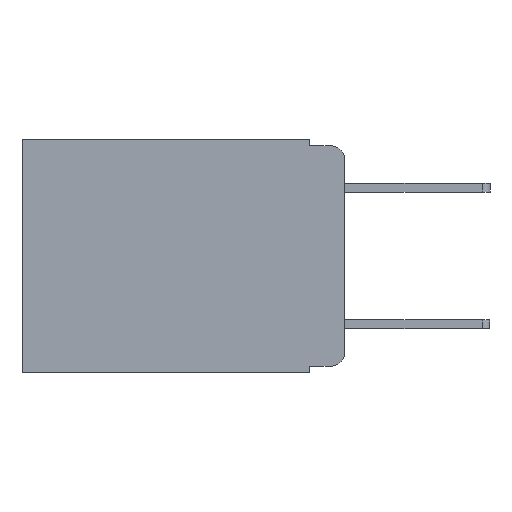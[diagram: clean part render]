
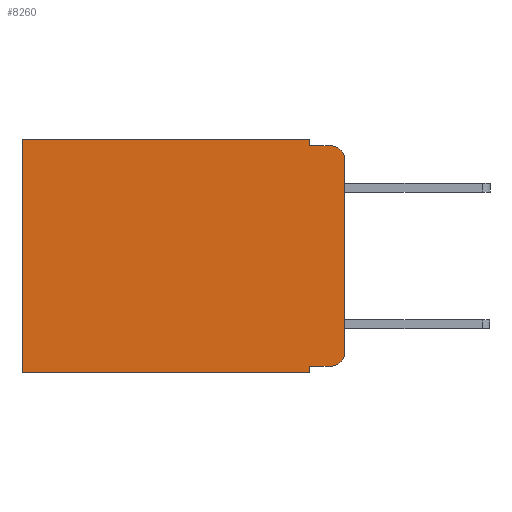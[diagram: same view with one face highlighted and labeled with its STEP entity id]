
A CAD part, left-side view. The second image highlights one B-rep face of the part: STEP entity #8260.
In plain terms, the highlighted planar face has unit normal (-1, 0, 0).
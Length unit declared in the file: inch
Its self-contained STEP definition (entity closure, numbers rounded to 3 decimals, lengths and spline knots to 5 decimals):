
#96 = CARTESIAN_POINT ( 'NONE',  ( 0.298, 0.051, -0.333 ) ) ;
#191 = ORIENTED_EDGE ( 'NONE', *, *, #8886, .T. ) ;
#301 = CARTESIAN_POINT ( 'NONE',  ( 0.298, 0.02, -0.01 ) ) ;
#340 = VECTOR ( 'NONE', #5273, 39.37008 ) ;
#369 = ORIENTED_EDGE ( 'NONE', *, *, #5522, .F. ) ;
#447 = CARTESIAN_POINT ( 'NONE',  ( 0.298, 0.051, -0.01 ) ) ;
#475 = EDGE_CURVE ( 'NONE', #3804, #5136, #2116, .T. ) ;
#532 = ORIENTED_EDGE ( 'NONE', *, *, #4509, .F. ) ;
#553 = DIRECTION ( 'NONE',  ( 0., 1., 0. ) ) ;
#648 = ORIENTED_EDGE ( 'NONE', *, *, #6500, .F. ) ;
#670 = ORIENTED_EDGE ( 'NONE', *, *, #9813, .F. ) ;
#727 = CARTESIAN_POINT ( 'NONE',  ( 0.298, 0.051, -0.343 ) ) ;
#878 = AXIS2_PLACEMENT_3D ( 'NONE', #7612, #3072, #8315 ) ;
#891 = ORIENTED_EDGE ( 'NONE', *, *, #475, .T. ) ;
#930 = CARTESIAN_POINT ( 'NONE',  ( 0.298, 0., 0. ) ) ;
#1177 = ORIENTED_EDGE ( 'NONE', *, *, #3389, .T. ) ;
#1271 = VERTEX_POINT ( 'NONE', #3354 ) ;
#1508 = DIRECTION ( 'NONE',  ( 1., 0., 0. ) ) ;
#1800 = VECTOR ( 'NONE', #7991, 39.37008 ) ;
#1916 = LINE ( 'NONE', #930, #5602 ) ;
#1981 = CARTESIAN_POINT ( 'NONE',  ( 0.298, 0.051, 0. ) ) ;
#2116 = LINE ( 'NONE', #6497, #6000 ) ;
#2119 = FACE_OUTER_BOUND ( 'NONE', #6079, .T. ) ;
#2330 = DIRECTION ( 'NONE',  ( 0., 0., -1. ) ) ;
#2523 = VERTEX_POINT ( 'NONE', #1981 ) ;
#2611 = EDGE_CURVE ( 'NONE', #2523, #4865, #4943, .T. ) ;
#3072 = DIRECTION ( 'NONE',  ( -1., 0., 0. ) ) ;
#3354 = CARTESIAN_POINT ( 'NONE',  ( 0.298, 0., -0.03 ) ) ;
#3389 = EDGE_CURVE ( 'NONE', #5136, #4146, #3807, .T. ) ;
#3478 = ORIENTED_EDGE ( 'NONE', *, *, #2611, .T. ) ;
#3757 = CARTESIAN_POINT ( 'NONE',  ( 0.298, 0., -0.313 ) ) ;
#3804 = VERTEX_POINT ( 'NONE', #96 ) ;
#3807 = CIRCLE ( 'NONE', #6703, 0.02 ) ;
#3813 = CARTESIAN_POINT ( 'NONE',  ( 0.298, 0., 0. ) ) ;
#3860 = VECTOR ( 'NONE', #2330, 39.37008 ) ;
#3902 = CARTESIAN_POINT ( 'NONE',  ( 0.298, 0., 0. ) ) ;
#3984 = DIRECTION ( 'NONE',  ( 0., 0., -1. ) ) ;
#4146 = VERTEX_POINT ( 'NONE', #3757 ) ;
#4348 = CARTESIAN_POINT ( 'NONE',  ( 0.298, 0.051, 0. ) ) ;
#4353 = VERTEX_POINT ( 'NONE', #727 ) ;
#4406 = VERTEX_POINT ( 'NONE', #8168 ) ;
#4509 = EDGE_CURVE ( 'NONE', #4353, #4406, #9708, .T. ) ;
#4544 = DIRECTION ( 'NONE',  ( 0., -1., 0. ) ) ;
#4656 = CARTESIAN_POINT ( 'NONE',  ( 0.298, 0.051, 0. ) ) ;
#4662 = EDGE_CURVE ( 'NONE', #1271, #4146, #1916, .T. ) ;
#4811 = CARTESIAN_POINT ( 'NONE',  ( 0.298, 0.02, -0.333 ) ) ;
#4865 = VERTEX_POINT ( 'NONE', #5964 ) ;
#4943 = LINE ( 'NONE', #3813, #340 ) ;
#5031 = EDGE_CURVE ( 'NONE', #1271, #9336, #8971, .T. ) ;
#5136 = VERTEX_POINT ( 'NONE', #4811 ) ;
#5247 = AXIS2_PLACEMENT_3D ( 'NONE', #3902, #1508, #6920 ) ;
#5260 = CARTESIAN_POINT ( 'NONE',  ( 0.298, 0.02, -0.313 ) ) ;
#5273 = DIRECTION ( 'NONE',  ( 0., 1., 0. ) ) ;
#5354 = CARTESIAN_POINT ( 'NONE',  ( 0.298, 0., -0.343 ) ) ;
#5522 = EDGE_CURVE ( 'NONE', #9002, #9336, #7095, .T. ) ;
#5602 = VECTOR ( 'NONE', #9237, 39.37008 ) ;
#5614 = DIRECTION ( 'NONE',  ( 0., -1., 0. ) ) ;
#5964 = CARTESIAN_POINT ( 'NONE',  ( 0.298, 0.473, 0. ) ) ;
#6000 = VECTOR ( 'NONE', #5614, 39.37008 ) ;
#6008 = ORIENTED_EDGE ( 'NONE', *, *, #5031, .T. ) ;
#6079 = EDGE_LOOP ( 'NONE', ( #7173, #6008, #369, #648, #3478, #191, #532, #670, #891, #1177 ) ) ;
#6111 = LINE ( 'NONE', #6907, #3860 ) ;
#6165 = VECTOR ( 'NONE', #553, 39.37008 ) ;
#6497 = CARTESIAN_POINT ( 'NONE',  ( 0.298, 0.051, -0.333 ) ) ;
#6500 = EDGE_CURVE ( 'NONE', #2523, #9002, #9700, .T. ) ;
#6657 = VECTOR ( 'NONE', #8291, 39.37008 ) ;
#6703 = AXIS2_PLACEMENT_3D ( 'NONE', #5260, #9147, #3984 ) ;
#6883 = LINE ( 'NONE', #4656, #6657 ) ;
#6889 = PLANE ( 'NONE',  #5247 ) ;
#6907 = CARTESIAN_POINT ( 'NONE',  ( 0.298, 0.473, 0. ) ) ;
#6920 = DIRECTION ( 'NONE',  ( 0., 0., -1. ) ) ;
#7095 = LINE ( 'NONE', #447, #8743 ) ;
#7173 = ORIENTED_EDGE ( 'NONE', *, *, #4662, .F. ) ;
#7612 = CARTESIAN_POINT ( 'NONE',  ( 0.298, 0.02, -0.03 ) ) ;
#7781 = CARTESIAN_POINT ( 'NONE',  ( 0.298, 0.051, -0.01 ) ) ;
#7991 = DIRECTION ( 'NONE',  ( 0., 0., -1. ) ) ;
#8168 = CARTESIAN_POINT ( 'NONE',  ( 0.298, 0.473, -0.343 ) ) ;
#8260 = ADVANCED_FACE ( 'NONE', ( #2119 ), #6889, .F. ) ;
#8291 = DIRECTION ( 'NONE',  ( 0., 0., -1. ) ) ;
#8315 = DIRECTION ( 'NONE',  ( 0., 0., -1. ) ) ;
#8743 = VECTOR ( 'NONE', #4544, 39.37008 ) ;
#8886 = EDGE_CURVE ( 'NONE', #4865, #4406, #6111, .T. ) ;
#8971 = CIRCLE ( 'NONE', #878, 0.02 ) ;
#9002 = VERTEX_POINT ( 'NONE', #7781 ) ;
#9147 = DIRECTION ( 'NONE',  ( -1., 0., 0. ) ) ;
#9237 = DIRECTION ( 'NONE',  ( 0., 0., -1. ) ) ;
#9336 = VERTEX_POINT ( 'NONE', #301 ) ;
#9700 = LINE ( 'NONE', #4348, #1800 ) ;
#9708 = LINE ( 'NONE', #5354, #6165 ) ;
#9813 = EDGE_CURVE ( 'NONE', #3804, #4353, #6883, .T. ) ;
